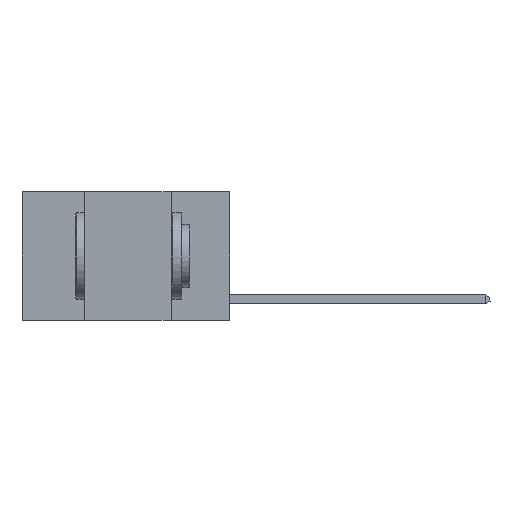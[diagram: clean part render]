
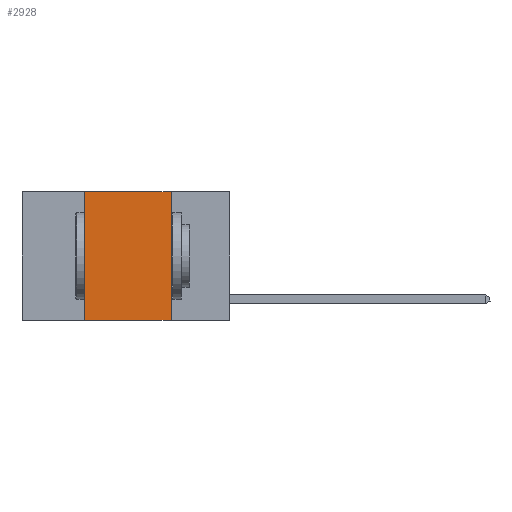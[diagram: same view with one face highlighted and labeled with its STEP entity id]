
A CAD part, left-side view. The second image highlights one B-rep face of the part: STEP entity #2928.
In plain terms, the highlighted planar face has unit normal (-1, 0, 0).
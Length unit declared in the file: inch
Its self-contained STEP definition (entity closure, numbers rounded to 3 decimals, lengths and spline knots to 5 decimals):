
#37 = DIRECTION ( 'NONE',  ( 0., 0., -1. ) ) ;
#148 = DIRECTION ( 'NONE',  ( 0., 0., 1. ) ) ;
#680 = EDGE_LOOP ( 'NONE', ( #12990, #2414, #13675, #16404 ) ) ;
#2217 = CARTESIAN_POINT ( 'NONE',  ( 0., 0.42, -0.37 ) ) ;
#2414 = ORIENTED_EDGE ( 'NONE', *, *, #2837, .F. ) ;
#2505 = EDGE_CURVE ( 'NONE', #4631, #10229, #6671, .T. ) ;
#2837 = EDGE_CURVE ( 'NONE', #6363, #4631, #4543, .T. ) ;
#2928 = ADVANCED_FACE ( 'NONE', ( #5340 ), #11811, .F. ) ;
#3251 = EDGE_CURVE ( 'NONE', #15946, #6363, #3715, .T. ) ;
#3311 = EDGE_CURVE ( 'NONE', #15946, #10229, #5789, .T. ) ;
#3409 = VECTOR ( 'NONE', #148, 39.37008 ) ;
#3715 = LINE ( 'NONE', #9490, #3409 ) ;
#3807 = AXIS2_PLACEMENT_3D ( 'NONE', #17232, #9175, #7944 ) ;
#4101 = VECTOR ( 'NONE', #9968, 39.37008 ) ;
#4543 = LINE ( 'NONE', #10238, #4101 ) ;
#4631 = VERTEX_POINT ( 'NONE', #15148 ) ;
#4855 = CARTESIAN_POINT ( 'NONE',  ( 0., 0.42, 0. ) ) ;
#5340 = FACE_OUTER_BOUND ( 'NONE', #680, .T. ) ;
#5789 = LINE ( 'NONE', #9944, #12783 ) ;
#6363 = VERTEX_POINT ( 'NONE', #4855 ) ;
#6671 = LINE ( 'NONE', #7987, #9541 ) ;
#7944 = DIRECTION ( 'NONE',  ( 0., 0., -1. ) ) ;
#7987 = CARTESIAN_POINT ( 'NONE',  ( 0., 0.17, 0. ) ) ;
#9175 = DIRECTION ( 'NONE',  ( 1., 0., 0. ) ) ;
#9490 = CARTESIAN_POINT ( 'NONE',  ( 0., 0.42, 0. ) ) ;
#9541 = VECTOR ( 'NONE', #37, 39.37008 ) ;
#9944 = CARTESIAN_POINT ( 'NONE',  ( 0., 0.6, -0.37 ) ) ;
#9968 = DIRECTION ( 'NONE',  ( 0., -1., 0. ) ) ;
#10229 = VERTEX_POINT ( 'NONE', #12072 ) ;
#10238 = CARTESIAN_POINT ( 'NONE',  ( 0., 0.6, 0. ) ) ;
#11811 = PLANE ( 'NONE',  #3807 ) ;
#12072 = CARTESIAN_POINT ( 'NONE',  ( 0., 0.17, -0.37 ) ) ;
#12783 = VECTOR ( 'NONE', #16589, 39.37008 ) ;
#12990 = ORIENTED_EDGE ( 'NONE', *, *, #2505, .F. ) ;
#13675 = ORIENTED_EDGE ( 'NONE', *, *, #3251, .F. ) ;
#15148 = CARTESIAN_POINT ( 'NONE',  ( 0., 0.17, 0. ) ) ;
#15946 = VERTEX_POINT ( 'NONE', #2217 ) ;
#16404 = ORIENTED_EDGE ( 'NONE', *, *, #3311, .T. ) ;
#16589 = DIRECTION ( 'NONE',  ( 0., -1., 0. ) ) ;
#17232 = CARTESIAN_POINT ( 'NONE',  ( 0., 0.6, 0. ) ) ;
